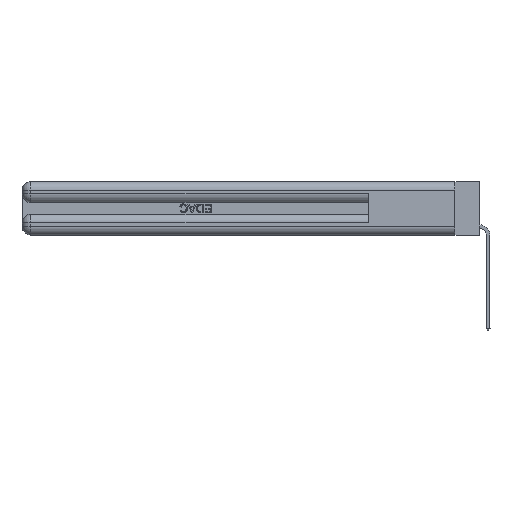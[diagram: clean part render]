
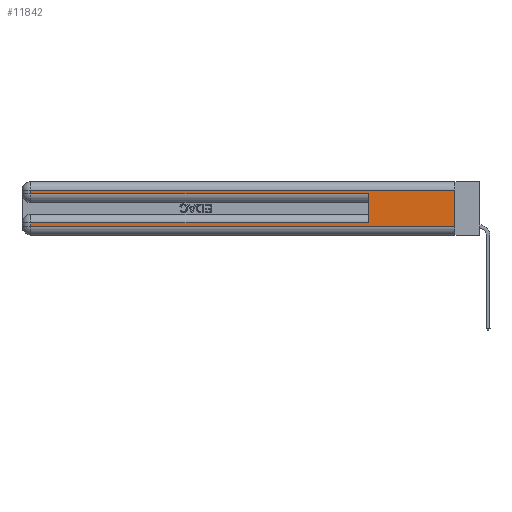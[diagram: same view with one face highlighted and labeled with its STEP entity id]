
A CAD part, left-side view. The second image highlights one B-rep face of the part: STEP entity #11842.
In plain terms, the highlighted planar face has unit normal (-1, 0, 0).
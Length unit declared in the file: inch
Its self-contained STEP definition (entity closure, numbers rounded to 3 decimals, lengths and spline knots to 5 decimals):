
#428 = EDGE_CURVE ( 'NONE', #8809, #24894, #6506, .T. ) ;
#444 = DIRECTION ( 'NONE',  ( 0., 1., 0. ) ) ;
#843 = LINE ( 'NONE', #5182, #10825 ) ;
#983 = VECTOR ( 'NONE', #6422, 39.37008 ) ;
#1080 = VERTEX_POINT ( 'NONE', #22772 ) ;
#1429 = VERTEX_POINT ( 'NONE', #27434 ) ;
#1526 = VECTOR ( 'NONE', #10294, 39.37008 ) ;
#1926 = AXIS2_PLACEMENT_3D ( 'NONE', #10913, #25834, #13062 ) ;
#2760 = DIRECTION ( 'NONE',  ( 0., 0., 1. ) ) ;
#3145 = EDGE_CURVE ( 'NONE', #14793, #1080, #16456, .T. ) ;
#3684 = CARTESIAN_POINT ( 'NONE',  ( 0., 2.94, 0.285 ) ) ;
#3812 = LINE ( 'NONE', #15256, #25818 ) ;
#4288 = CARTESIAN_POINT ( 'NONE',  ( 0., 0., 0.06 ) ) ;
#4441 = VECTOR ( 'NONE', #14385, 39.37008 ) ;
#4487 = PLANE ( 'NONE',  #1926 ) ;
#4865 = CARTESIAN_POINT ( 'NONE',  ( 0., 2.94, 0.37 ) ) ;
#4879 = CARTESIAN_POINT ( 'NONE',  ( 0., 0.6, 0.145 ) ) ;
#5182 = CARTESIAN_POINT ( 'NONE',  ( 0., 0., 0.37 ) ) ;
#6300 = CARTESIAN_POINT ( 'NONE',  ( 0., 0., 0.31 ) ) ;
#6316 = EDGE_CURVE ( 'NONE', #24894, #15767, #24340, .T. ) ;
#6422 = DIRECTION ( 'NONE',  ( 0., -1., 0. ) ) ;
#6506 = LINE ( 'NONE', #20947, #1526 ) ;
#6662 = LINE ( 'NONE', #4879, #22357 ) ;
#7010 = DIRECTION ( 'NONE',  ( 0., 0., -1. ) ) ;
#7320 = DIRECTION ( 'NONE',  ( 0., 0., -1. ) ) ;
#7936 = CARTESIAN_POINT ( 'NONE',  ( 0., 0., 0.285 ) ) ;
#8100 = CARTESIAN_POINT ( 'NONE',  ( 0., 2.94, 0.06 ) ) ;
#8809 = VERTEX_POINT ( 'NONE', #14620 ) ;
#9505 = VECTOR ( 'NONE', #7010, 39.37008 ) ;
#10016 = ORIENTED_EDGE ( 'NONE', *, *, #6316, .T. ) ;
#10294 = DIRECTION ( 'NONE',  ( 0., 0., -1. ) ) ;
#10724 = EDGE_CURVE ( 'NONE', #18929, #15767, #843, .T. ) ;
#10825 = VECTOR ( 'NONE', #7320, 39.37008 ) ;
#10913 = CARTESIAN_POINT ( 'NONE',  ( 0., 0., 0.37 ) ) ;
#11220 = EDGE_CURVE ( 'NONE', #15459, #8809, #3812, .T. ) ;
#11842 = ADVANCED_FACE ( 'NONE', ( #16114 ), #4487, .F. ) ;
#13062 = DIRECTION ( 'NONE',  ( 0., 0., -1. ) ) ;
#13081 = ORIENTED_EDGE ( 'NONE', *, *, #25234, .T. ) ;
#13863 = ORIENTED_EDGE ( 'NONE', *, *, #428, .T. ) ;
#14168 = CARTESIAN_POINT ( 'NONE',  ( 0., 0.6, 0.085 ) ) ;
#14385 = DIRECTION ( 'NONE',  ( 0., -1., 0. ) ) ;
#14620 = CARTESIAN_POINT ( 'NONE',  ( 0., 2.94, 0.085 ) ) ;
#14793 = VERTEX_POINT ( 'NONE', #3684 ) ;
#15256 = CARTESIAN_POINT ( 'NONE',  ( 0., 0., 0.085 ) ) ;
#15459 = VERTEX_POINT ( 'NONE', #14168 ) ;
#15581 = DIRECTION ( 'NONE',  ( 0., 1., 0. ) ) ;
#15767 = VERTEX_POINT ( 'NONE', #25816 ) ;
#16114 = FACE_OUTER_BOUND ( 'NONE', #21067, .T. ) ;
#16452 = ORIENTED_EDGE ( 'NONE', *, *, #22059, .T. ) ;
#16456 = LINE ( 'NONE', #7936, #4441 ) ;
#17164 = ORIENTED_EDGE ( 'NONE', *, *, #11220, .T. ) ;
#17723 = ORIENTED_EDGE ( 'NONE', *, *, #3145, .T. ) ;
#18154 = EDGE_CURVE ( 'NONE', #15459, #1080, #6662, .T. ) ;
#18929 = VERTEX_POINT ( 'NONE', #6300 ) ;
#20947 = CARTESIAN_POINT ( 'NONE',  ( 0., 2.94, 0.37 ) ) ;
#21067 = EDGE_LOOP ( 'NONE', ( #24919, #13081, #16452, #17723, #26912, #17164, #13863, #10016 ) ) ;
#21921 = CARTESIAN_POINT ( 'NONE',  ( 0., 0., 0.31 ) ) ;
#22059 = EDGE_CURVE ( 'NONE', #1429, #14793, #26528, .T. ) ;
#22357 = VECTOR ( 'NONE', #2760, 39.37008 ) ;
#22772 = CARTESIAN_POINT ( 'NONE',  ( 0., 0.6, 0.285 ) ) ;
#24340 = LINE ( 'NONE', #4288, #983 ) ;
#24392 = LINE ( 'NONE', #21921, #25052 ) ;
#24894 = VERTEX_POINT ( 'NONE', #8100 ) ;
#24919 = ORIENTED_EDGE ( 'NONE', *, *, #10724, .F. ) ;
#25052 = VECTOR ( 'NONE', #15581, 39.37008 ) ;
#25234 = EDGE_CURVE ( 'NONE', #18929, #1429, #24392, .T. ) ;
#25816 = CARTESIAN_POINT ( 'NONE',  ( 0., 0., 0.06 ) ) ;
#25818 = VECTOR ( 'NONE', #444, 39.37008 ) ;
#25834 = DIRECTION ( 'NONE',  ( 1., 0., 0. ) ) ;
#26528 = LINE ( 'NONE', #4865, #9505 ) ;
#26912 = ORIENTED_EDGE ( 'NONE', *, *, #18154, .F. ) ;
#27434 = CARTESIAN_POINT ( 'NONE',  ( 0., 2.94, 0.31 ) ) ;
